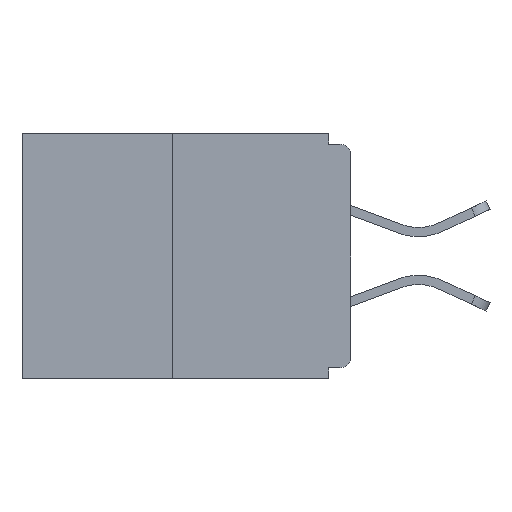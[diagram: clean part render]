
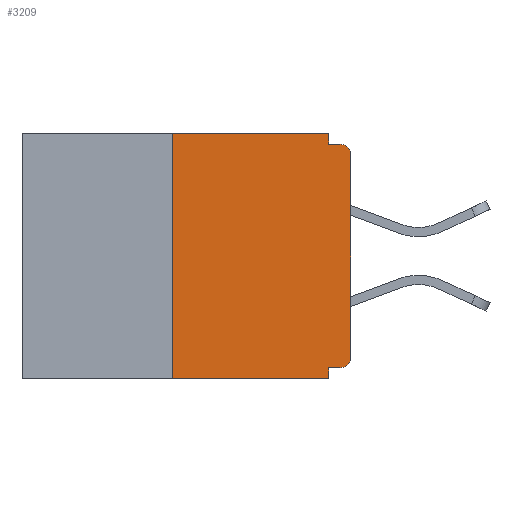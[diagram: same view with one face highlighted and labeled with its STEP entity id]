
A CAD part, left-side view. The second image highlights one B-rep face of the part: STEP entity #3209.
In plain terms, the highlighted planar face has unit normal (-1, 0, 0).
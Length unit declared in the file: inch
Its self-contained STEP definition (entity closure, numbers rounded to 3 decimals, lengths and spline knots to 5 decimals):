
#209 = CARTESIAN_POINT ( 'NONE',  ( 0., 0.25, -0.343 ) ) ;
#727 = VERTEX_POINT ( 'NONE', #10726 ) ;
#740 = VECTOR ( 'NONE', #7672, 39.37008 ) ;
#1005 = ORIENTED_EDGE ( 'NONE', *, *, #11467, .F. ) ;
#1083 = DIRECTION ( 'NONE',  ( 0., 0., -1. ) ) ;
#1452 = ORIENTED_EDGE ( 'NONE', *, *, #6514, .T. ) ;
#1838 = VECTOR ( 'NONE', #12811, 39.37008 ) ;
#2047 = CARTESIAN_POINT ( 'NONE',  ( 0., 0.015, -0.328 ) ) ;
#2075 = CARTESIAN_POINT ( 'NONE',  ( 0., 0., -0.015 ) ) ;
#2233 = PLANE ( 'NONE',  #11478 ) ;
#2645 = ORIENTED_EDGE ( 'NONE', *, *, #8626, .F. ) ;
#2772 = DIRECTION ( 'NONE',  ( 0., 0., 1. ) ) ;
#3077 = VERTEX_POINT ( 'NONE', #209 ) ;
#3209 = ADVANCED_FACE ( 'NONE', ( #3764 ), #2233, .F. ) ;
#3281 = CARTESIAN_POINT ( 'NONE',  ( 0., 0.031, 0. ) ) ;
#3653 = ORIENTED_EDGE ( 'NONE', *, *, #13413, .T. ) ;
#3702 = VECTOR ( 'NONE', #12199, 39.37008 ) ;
#3764 = FACE_OUTER_BOUND ( 'NONE', #8804, .T. ) ;
#4043 = ORIENTED_EDGE ( 'NONE', *, *, #9801, .F. ) ;
#4286 = EDGE_CURVE ( 'NONE', #7876, #727, #13546, .T. ) ;
#4297 = EDGE_CURVE ( 'NONE', #13679, #8217, #10670, .T. ) ;
#4410 = DIRECTION ( 'NONE',  ( 0., 0., -1. ) ) ;
#4833 = ORIENTED_EDGE ( 'NONE', *, *, #4297, .F. ) ;
#4918 = VECTOR ( 'NONE', #5720, 39.37008 ) ;
#5024 = CARTESIAN_POINT ( 'NONE',  ( 0., 0., -0.313 ) ) ;
#5061 = EDGE_CURVE ( 'NONE', #10820, #10947, #10308, .T. ) ;
#5463 = VECTOR ( 'NONE', #2772, 39.37008 ) ;
#5698 = VECTOR ( 'NONE', #6493, 39.37008 ) ;
#5720 = DIRECTION ( 'NONE',  ( 0., 1., 0. ) ) ;
#5941 = LINE ( 'NONE', #12896, #13883 ) ;
#6208 = CARTESIAN_POINT ( 'NONE',  ( 0., 0.46, 0. ) ) ;
#6479 = LINE ( 'NONE', #2075, #740 ) ;
#6493 = DIRECTION ( 'NONE',  ( 0., 0., 1. ) ) ;
#6514 = EDGE_CURVE ( 'NONE', #13679, #7835, #7566, .T. ) ;
#6771 = CARTESIAN_POINT ( 'NONE',  ( 0., 0., -0.03 ) ) ;
#6989 = EDGE_CURVE ( 'NONE', #3077, #13720, #9781, .T. ) ;
#7209 = EDGE_CURVE ( 'NONE', #3077, #12784, #13978, .T. ) ;
#7256 = ORIENTED_EDGE ( 'NONE', *, *, #7209, .F. ) ;
#7322 = CARTESIAN_POINT ( 'NONE',  ( 0., 0.031, -0.328 ) ) ;
#7346 = LINE ( 'NONE', #6208, #9048 ) ;
#7566 = CIRCLE ( 'NONE', #8778, 0.015 ) ;
#7578 = CARTESIAN_POINT ( 'NONE',  ( 0., 0.015, -0.03 ) ) ;
#7672 = DIRECTION ( 'NONE',  ( 0., -1., 0. ) ) ;
#7737 = ORIENTED_EDGE ( 'NONE', *, *, #5061, .F. ) ;
#7835 = VERTEX_POINT ( 'NONE', #5024 ) ;
#7876 = VERTEX_POINT ( 'NONE', #6771 ) ;
#7881 = CARTESIAN_POINT ( 'NONE',  ( 0., 0.015, -0.313 ) ) ;
#8217 = VERTEX_POINT ( 'NONE', #7322 ) ;
#8626 = EDGE_CURVE ( 'NONE', #12784, #10820, #7346, .T. ) ;
#8778 = AXIS2_PLACEMENT_3D ( 'NONE', #7881, #12107, #10113 ) ;
#8804 = EDGE_LOOP ( 'NONE', ( #2645, #7256, #9858, #1005, #4833, #1452, #3653, #12905, #4043, #7737 ) ) ;
#9048 = VECTOR ( 'NONE', #13640, 39.37008 ) ;
#9092 = CARTESIAN_POINT ( 'NONE',  ( 0., 0.25, 0. ) ) ;
#9770 = DIRECTION ( 'NONE',  ( 0., 0., -1. ) ) ;
#9772 = DIRECTION ( 'NONE',  ( -1., 0., 0. ) ) ;
#9781 = LINE ( 'NONE', #11503, #1838 ) ;
#9801 = EDGE_CURVE ( 'NONE', #10947, #727, #6479, .T. ) ;
#9858 = ORIENTED_EDGE ( 'NONE', *, *, #6989, .T. ) ;
#9889 = DIRECTION ( 'NONE',  ( 1., 0., 0. ) ) ;
#9963 = CARTESIAN_POINT ( 'NONE',  ( 0., 0.031, -0.015 ) ) ;
#10113 = DIRECTION ( 'NONE',  ( 0., 0., -1. ) ) ;
#10308 = LINE ( 'NONE', #11165, #3702 ) ;
#10670 = LINE ( 'NONE', #12204, #4918 ) ;
#10726 = CARTESIAN_POINT ( 'NONE',  ( 0., 0.015, -0.015 ) ) ;
#10820 = VERTEX_POINT ( 'NONE', #3281 ) ;
#10883 = CARTESIAN_POINT ( 'NONE',  ( 0., 0.46, 0. ) ) ;
#10947 = VERTEX_POINT ( 'NONE', #9963 ) ;
#11165 = CARTESIAN_POINT ( 'NONE',  ( 0., 0.031, 0. ) ) ;
#11467 = EDGE_CURVE ( 'NONE', #8217, #13720, #5941, .T. ) ;
#11478 = AXIS2_PLACEMENT_3D ( 'NONE', #10883, #9889, #4410 ) ;
#11503 = CARTESIAN_POINT ( 'NONE',  ( 0., 0.46, -0.343 ) ) ;
#11926 = AXIS2_PLACEMENT_3D ( 'NONE', #7578, #9772, #1083 ) ;
#12075 = CARTESIAN_POINT ( 'NONE',  ( 0., 0.25, 0. ) ) ;
#12107 = DIRECTION ( 'NONE',  ( -1., 0., 0. ) ) ;
#12199 = DIRECTION ( 'NONE',  ( 0., 0., -1. ) ) ;
#12204 = CARTESIAN_POINT ( 'NONE',  ( 0., 0., -0.328 ) ) ;
#12784 = VERTEX_POINT ( 'NONE', #9092 ) ;
#12811 = DIRECTION ( 'NONE',  ( 0., -1., 0. ) ) ;
#12896 = CARTESIAN_POINT ( 'NONE',  ( 0., 0.031, -0.343 ) ) ;
#12905 = ORIENTED_EDGE ( 'NONE', *, *, #4286, .T. ) ;
#13413 = EDGE_CURVE ( 'NONE', #7835, #7876, #13748, .T. ) ;
#13546 = CIRCLE ( 'NONE', #11926, 0.015 ) ;
#13562 = CARTESIAN_POINT ( 'NONE',  ( 0., 0., 0. ) ) ;
#13640 = DIRECTION ( 'NONE',  ( 0., -1., 0. ) ) ;
#13679 = VERTEX_POINT ( 'NONE', #2047 ) ;
#13720 = VERTEX_POINT ( 'NONE', #13895 ) ;
#13748 = LINE ( 'NONE', #13562, #5463 ) ;
#13883 = VECTOR ( 'NONE', #9770, 39.37008 ) ;
#13895 = CARTESIAN_POINT ( 'NONE',  ( 0., 0.031, -0.343 ) ) ;
#13978 = LINE ( 'NONE', #12075, #5698 ) ;
